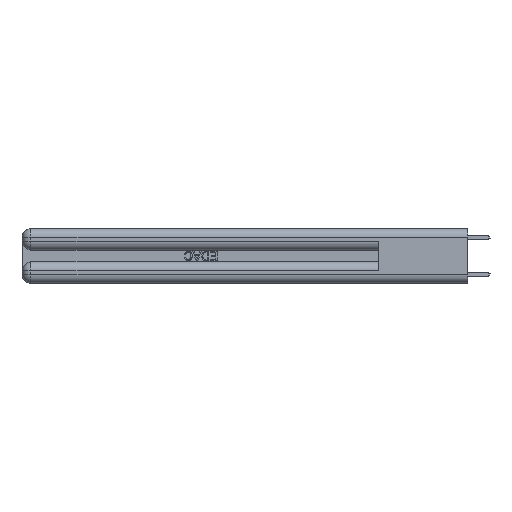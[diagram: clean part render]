
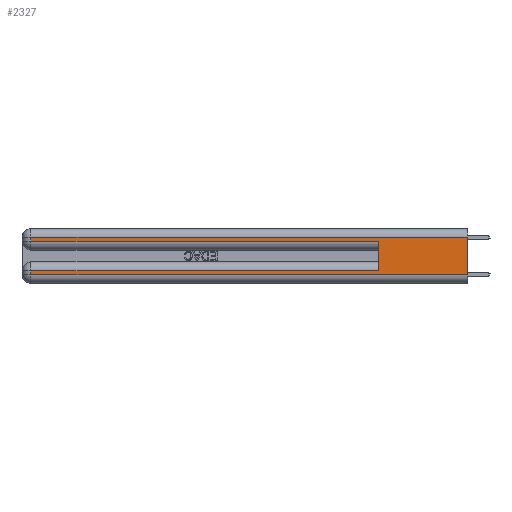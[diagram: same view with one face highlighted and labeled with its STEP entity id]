
A CAD part, left-side view. The second image highlights one B-rep face of the part: STEP entity #2327.
In plain terms, the highlighted planar face has unit normal (-1, 0, 0).
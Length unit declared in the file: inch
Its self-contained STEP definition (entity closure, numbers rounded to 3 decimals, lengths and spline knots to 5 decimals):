
#916 = CARTESIAN_POINT ( 'NONE',  ( 0., 0., 0.37 ) ) ;
#1297 = AXIS2_PLACEMENT_3D ( 'NONE', #916, #18200, #23566 ) ;
#1580 = VECTOR ( 'NONE', #8202, 39.37008 ) ;
#2022 = ORIENTED_EDGE ( 'NONE', *, *, #15388, .T. ) ;
#2206 = CARTESIAN_POINT ( 'NONE',  ( 0., 0., 0.31 ) ) ;
#2277 = VERTEX_POINT ( 'NONE', #16163 ) ;
#2327 = ADVANCED_FACE ( 'NONE', ( #23896 ), #13342, .F. ) ;
#4317 = CARTESIAN_POINT ( 'NONE',  ( 0., 0., 0.06 ) ) ;
#4622 = VECTOR ( 'NONE', #12892, 39.37008 ) ;
#4664 = EDGE_CURVE ( 'NONE', #21479, #25936, #5527, .T. ) ;
#5073 = EDGE_CURVE ( 'NONE', #6861, #30891, #10864, .T. ) ;
#5463 = CARTESIAN_POINT ( 'NONE',  ( 0., 0., 0.285 ) ) ;
#5527 = LINE ( 'NONE', #15762, #32939 ) ;
#6810 = CARTESIAN_POINT ( 'NONE',  ( 0., 0., 0.37 ) ) ;
#6861 = VERTEX_POINT ( 'NONE', #30658 ) ;
#6955 = EDGE_CURVE ( 'NONE', #18076, #2277, #18120, .T. ) ;
#7352 = VERTEX_POINT ( 'NONE', #18735 ) ;
#8202 = DIRECTION ( 'NONE',  ( 0., 0., -1. ) ) ;
#9151 = DIRECTION ( 'NONE',  ( 0., 0., -1. ) ) ;
#10702 = ORIENTED_EDGE ( 'NONE', *, *, #22339, .F. ) ;
#10864 = LINE ( 'NONE', #18249, #4622 ) ;
#11065 = VECTOR ( 'NONE', #13206, 39.37008 ) ;
#11921 = VECTOR ( 'NONE', #28011, 39.37008 ) ;
#12892 = DIRECTION ( 'NONE',  ( 0., -1., 0. ) ) ;
#13206 = DIRECTION ( 'NONE',  ( 0., -1., 0. ) ) ;
#13342 = PLANE ( 'NONE',  #1297 ) ;
#13390 = ORIENTED_EDGE ( 'NONE', *, *, #26547, .T. ) ;
#14411 = VECTOR ( 'NONE', #9151, 39.37008 ) ;
#14942 = LINE ( 'NONE', #2206, #11921 ) ;
#15388 = EDGE_CURVE ( 'NONE', #25630, #21479, #14942, .T. ) ;
#15762 = CARTESIAN_POINT ( 'NONE',  ( 0., 2.94, 0.37 ) ) ;
#15876 = VECTOR ( 'NONE', #17455, 39.37008 ) ;
#16163 = CARTESIAN_POINT ( 'NONE',  ( 0., 2.94, 0.085 ) ) ;
#16530 = CARTESIAN_POINT ( 'NONE',  ( 0., 0., 0.31 ) ) ;
#16703 = LINE ( 'NONE', #6810, #14411 ) ;
#17094 = ORIENTED_EDGE ( 'NONE', *, *, #28397, .F. ) ;
#17455 = DIRECTION ( 'NONE',  ( 0., 1., 0. ) ) ;
#18062 = DIRECTION ( 'NONE',  ( 0., 0., 1. ) ) ;
#18076 = VERTEX_POINT ( 'NONE', #31569 ) ;
#18120 = LINE ( 'NONE', #19968, #15876 ) ;
#18200 = DIRECTION ( 'NONE',  ( 1., 0., 0. ) ) ;
#18249 = CARTESIAN_POINT ( 'NONE',  ( 0., 0., 0.06 ) ) ;
#18735 = CARTESIAN_POINT ( 'NONE',  ( 0., 0.6, 0.285 ) ) ;
#18796 = ORIENTED_EDGE ( 'NONE', *, *, #6955, .T. ) ;
#19968 = CARTESIAN_POINT ( 'NONE',  ( 0., 0., 0.085 ) ) ;
#21204 = EDGE_CURVE ( 'NONE', #25936, #7352, #28442, .T. ) ;
#21479 = VERTEX_POINT ( 'NONE', #30195 ) ;
#22339 = EDGE_CURVE ( 'NONE', #18076, #7352, #25759, .T. ) ;
#23566 = DIRECTION ( 'NONE',  ( 0., 0., -1. ) ) ;
#23896 = FACE_OUTER_BOUND ( 'NONE', #23931, .T. ) ;
#23931 = EDGE_LOOP ( 'NONE', ( #17094, #2022, #29236, #29062, #10702, #18796, #13390, #28150 ) ) ;
#25599 = CARTESIAN_POINT ( 'NONE',  ( 0., 0.6, 0.145 ) ) ;
#25630 = VERTEX_POINT ( 'NONE', #16530 ) ;
#25759 = LINE ( 'NONE', #25599, #27087 ) ;
#25936 = VERTEX_POINT ( 'NONE', #30092 ) ;
#26547 = EDGE_CURVE ( 'NONE', #2277, #6861, #31639, .T. ) ;
#27087 = VECTOR ( 'NONE', #18062, 39.37008 ) ;
#28011 = DIRECTION ( 'NONE',  ( 0., 1., 0. ) ) ;
#28150 = ORIENTED_EDGE ( 'NONE', *, *, #5073, .T. ) ;
#28397 = EDGE_CURVE ( 'NONE', #25630, #30891, #16703, .T. ) ;
#28442 = LINE ( 'NONE', #5463, #11065 ) ;
#29062 = ORIENTED_EDGE ( 'NONE', *, *, #21204, .T. ) ;
#29236 = ORIENTED_EDGE ( 'NONE', *, *, #4664, .T. ) ;
#30092 = CARTESIAN_POINT ( 'NONE',  ( 0., 2.94, 0.285 ) ) ;
#30195 = CARTESIAN_POINT ( 'NONE',  ( 0., 2.94, 0.31 ) ) ;
#30658 = CARTESIAN_POINT ( 'NONE',  ( 0., 2.94, 0.06 ) ) ;
#30891 = VERTEX_POINT ( 'NONE', #4317 ) ;
#31156 = DIRECTION ( 'NONE',  ( 0., 0., -1. ) ) ;
#31477 = CARTESIAN_POINT ( 'NONE',  ( 0., 2.94, 0.37 ) ) ;
#31569 = CARTESIAN_POINT ( 'NONE',  ( 0., 0.6, 0.085 ) ) ;
#31639 = LINE ( 'NONE', #31477, #1580 ) ;
#32939 = VECTOR ( 'NONE', #31156, 39.37008 ) ;
